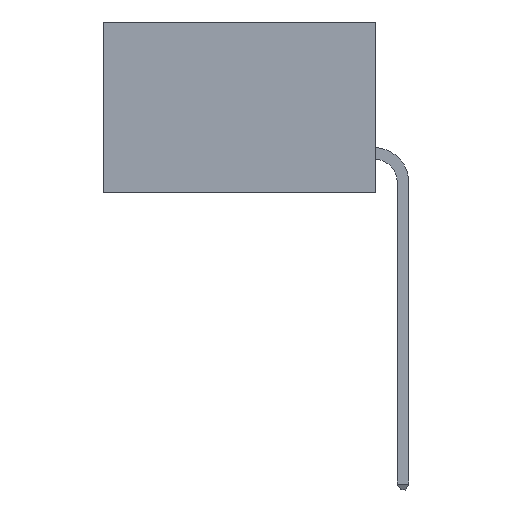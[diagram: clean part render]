
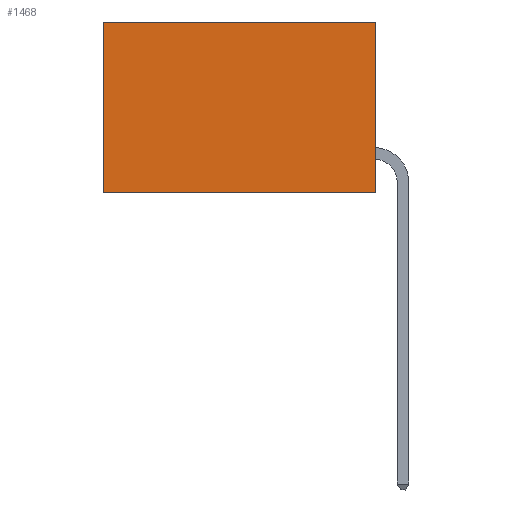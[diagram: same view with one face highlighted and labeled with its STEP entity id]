
A CAD part, left-side view. The second image highlights one B-rep face of the part: STEP entity #1468.
In plain terms, the highlighted planar face has unit normal (-1, 0, 0).
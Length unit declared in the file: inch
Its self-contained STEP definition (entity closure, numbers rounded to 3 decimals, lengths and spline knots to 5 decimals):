
#178 = VECTOR ( 'NONE', #6867, 39.37008 ) ;
#257 = CARTESIAN_POINT ( 'NONE',  ( 0.277, 0., -0.37 ) ) ;
#317 = DIRECTION ( 'NONE',  ( 1., 0., 0. ) ) ;
#362 = VECTOR ( 'NONE', #2806, 39.37008 ) ;
#973 = DIRECTION ( 'NONE',  ( 0., 0., -1. ) ) ;
#1409 = EDGE_CURVE ( 'NONE', #2436, #5299, #7932, .T. ) ;
#1468 = ADVANCED_FACE ( 'NONE', ( #3610 ), #1685, .F. ) ;
#1678 = ORIENTED_EDGE ( 'NONE', *, *, #6596, .F. ) ;
#1685 = PLANE ( 'NONE',  #3623 ) ;
#2209 = LINE ( 'NONE', #5410, #178 ) ;
#2325 = EDGE_CURVE ( 'NONE', #4468, #2436, #4397, .T. ) ;
#2436 = VERTEX_POINT ( 'NONE', #7263 ) ;
#2806 = DIRECTION ( 'NONE',  ( 0., 1., 0. ) ) ;
#3119 = VECTOR ( 'NONE', #4866, 39.37008 ) ;
#3604 = CARTESIAN_POINT ( 'NONE',  ( 0.277, 0., 0. ) ) ;
#3610 = FACE_OUTER_BOUND ( 'NONE', #6384, .T. ) ;
#3623 = AXIS2_PLACEMENT_3D ( 'NONE', #257, #317, #973 ) ;
#4166 = CARTESIAN_POINT ( 'NONE',  ( 0.277, 0., -0.37 ) ) ;
#4397 = LINE ( 'NONE', #5173, #362 ) ;
#4468 = VERTEX_POINT ( 'NONE', #3604 ) ;
#4800 = LINE ( 'NONE', #5899, #7516 ) ;
#4859 = CARTESIAN_POINT ( 'NONE',  ( 0.277, 0.59, -0.37 ) ) ;
#4866 = DIRECTION ( 'NONE',  ( 0., 0., -1. ) ) ;
#5173 = CARTESIAN_POINT ( 'NONE',  ( 0.277, 0., 0. ) ) ;
#5299 = VERTEX_POINT ( 'NONE', #7162 ) ;
#5410 = CARTESIAN_POINT ( 'NONE',  ( 0.277, 0., -0.37 ) ) ;
#5888 = DIRECTION ( 'NONE',  ( 0., 1., 0. ) ) ;
#5899 = CARTESIAN_POINT ( 'NONE',  ( 0.277, 0., -0.37 ) ) ;
#6384 = EDGE_LOOP ( 'NONE', ( #7825, #1678, #6708, #7956 ) ) ;
#6596 = EDGE_CURVE ( 'NONE', #7211, #5299, #4800, .T. ) ;
#6708 = ORIENTED_EDGE ( 'NONE', *, *, #6802, .F. ) ;
#6802 = EDGE_CURVE ( 'NONE', #4468, #7211, #2209, .T. ) ;
#6867 = DIRECTION ( 'NONE',  ( 0., 0., -1. ) ) ;
#7162 = CARTESIAN_POINT ( 'NONE',  ( 0.277, 0.59, -0.37 ) ) ;
#7211 = VERTEX_POINT ( 'NONE', #4166 ) ;
#7263 = CARTESIAN_POINT ( 'NONE',  ( 0.277, 0.59, 0. ) ) ;
#7516 = VECTOR ( 'NONE', #5888, 39.37008 ) ;
#7825 = ORIENTED_EDGE ( 'NONE', *, *, #1409, .T. ) ;
#7932 = LINE ( 'NONE', #4859, #3119 ) ;
#7956 = ORIENTED_EDGE ( 'NONE', *, *, #2325, .T. ) ;
